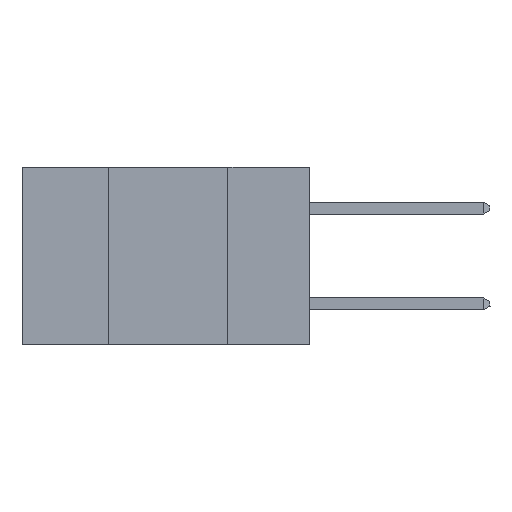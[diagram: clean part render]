
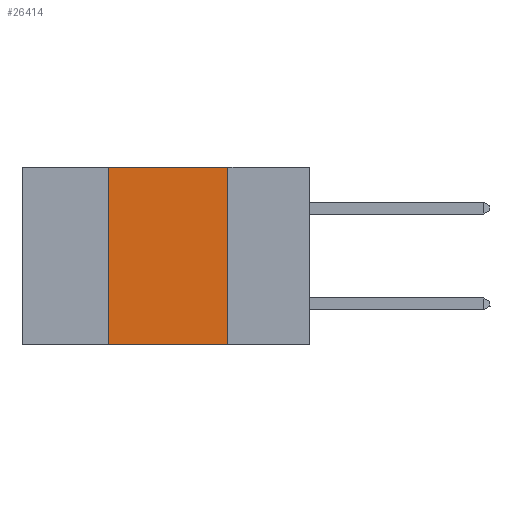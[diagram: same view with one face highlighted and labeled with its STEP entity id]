
A CAD part, left-side view. The second image highlights one B-rep face of the part: STEP entity #26414.
In plain terms, the highlighted planar face has unit normal (-1, 0, 0).
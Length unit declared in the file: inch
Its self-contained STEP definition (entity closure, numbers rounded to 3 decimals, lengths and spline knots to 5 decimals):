
#307 = CARTESIAN_POINT ( 'NONE',  ( 0., 0.42, 0. ) ) ;
#899 = LINE ( 'NONE', #17447, #21805 ) ;
#2580 = EDGE_LOOP ( 'NONE', ( #17604, #12200, #7179, #13034 ) ) ;
#2658 = VECTOR ( 'NONE', #18615, 39.37008 ) ;
#2819 = DIRECTION ( 'NONE',  ( 1., 0., 0. ) ) ;
#3570 = LINE ( 'NONE', #17783, #17437 ) ;
#4178 = EDGE_CURVE ( 'NONE', #4399, #22104, #899, .T. ) ;
#4399 = VERTEX_POINT ( 'NONE', #8985 ) ;
#5058 = EDGE_CURVE ( 'NONE', #4399, #21745, #3570, .T. ) ;
#5168 = DIRECTION ( 'NONE',  ( 0., 0., -1. ) ) ;
#5962 = CARTESIAN_POINT ( 'NONE',  ( 0., 0.17, 0. ) ) ;
#7141 = CARTESIAN_POINT ( 'NONE',  ( 0., 0.6, 0. ) ) ;
#7179 = ORIENTED_EDGE ( 'NONE', *, *, #4178, .F. ) ;
#8805 = VERTEX_POINT ( 'NONE', #5962 ) ;
#8985 = CARTESIAN_POINT ( 'NONE',  ( 0., 0.42, -0.37 ) ) ;
#9108 = PLANE ( 'NONE',  #11267 ) ;
#9290 = DIRECTION ( 'NONE',  ( 0., 0., 1. ) ) ;
#9884 = DIRECTION ( 'NONE',  ( 0., -1., 0. ) ) ;
#11267 = AXIS2_PLACEMENT_3D ( 'NONE', #7141, #2819, #5168 ) ;
#11668 = FACE_OUTER_BOUND ( 'NONE', #2580, .T. ) ;
#12200 = ORIENTED_EDGE ( 'NONE', *, *, #17154, .F. ) ;
#13034 = ORIENTED_EDGE ( 'NONE', *, *, #5058, .T. ) ;
#15085 = DIRECTION ( 'NONE',  ( 0., 0., -1. ) ) ;
#15365 = CARTESIAN_POINT ( 'NONE',  ( 0., 0.17, -0.37 ) ) ;
#15784 = LINE ( 'NONE', #23635, #17405 ) ;
#17154 = EDGE_CURVE ( 'NONE', #22104, #8805, #19388, .T. ) ;
#17405 = VECTOR ( 'NONE', #15085, 39.37008 ) ;
#17437 = VECTOR ( 'NONE', #9884, 39.37008 ) ;
#17447 = CARTESIAN_POINT ( 'NONE',  ( 0., 0.42, 0. ) ) ;
#17604 = ORIENTED_EDGE ( 'NONE', *, *, #23420, .F. ) ;
#17783 = CARTESIAN_POINT ( 'NONE',  ( 0., 0.6, -0.37 ) ) ;
#18615 = DIRECTION ( 'NONE',  ( 0., -1., 0. ) ) ;
#19388 = LINE ( 'NONE', #22585, #2658 ) ;
#21745 = VERTEX_POINT ( 'NONE', #15365 ) ;
#21805 = VECTOR ( 'NONE', #9290, 39.37008 ) ;
#22104 = VERTEX_POINT ( 'NONE', #307 ) ;
#22585 = CARTESIAN_POINT ( 'NONE',  ( 0., 0.6, 0. ) ) ;
#23420 = EDGE_CURVE ( 'NONE', #8805, #21745, #15784, .T. ) ;
#23635 = CARTESIAN_POINT ( 'NONE',  ( 0., 0.17, 0. ) ) ;
#26414 = ADVANCED_FACE ( 'NONE', ( #11668 ), #9108, .F. ) ;
